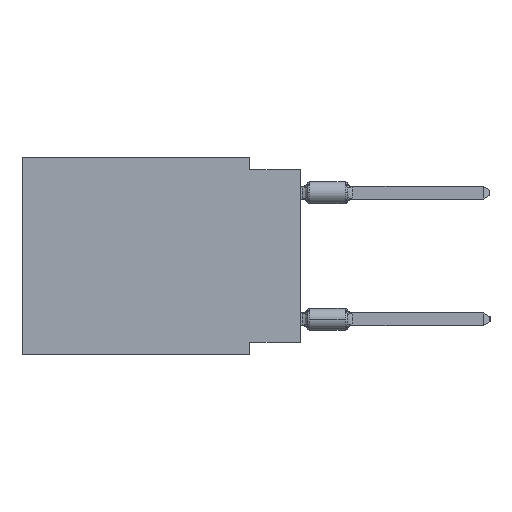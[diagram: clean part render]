
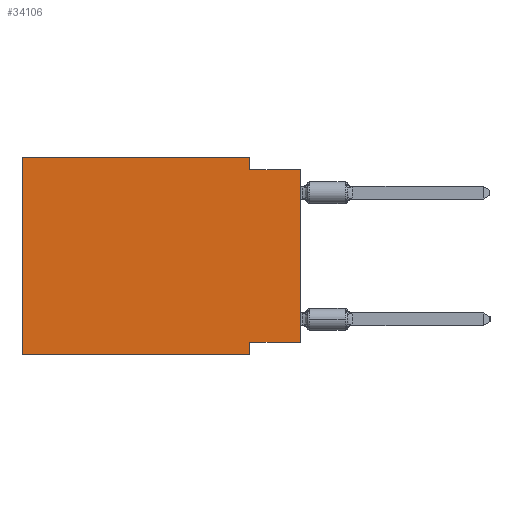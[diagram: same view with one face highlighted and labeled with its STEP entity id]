
A CAD part, left-side view. The second image highlights one B-rep face of the part: STEP entity #34106.
In plain terms, the highlighted planar face has unit normal (-1, 0, 0).
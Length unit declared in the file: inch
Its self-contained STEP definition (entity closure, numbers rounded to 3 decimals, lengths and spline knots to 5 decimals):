
#138 = EDGE_CURVE ( 'NONE', #9546, #27398, #3173, .T. ) ;
#613 = CARTESIAN_POINT ( 'NONE',  ( 0., 0., -0.365 ) ) ;
#2418 = DIRECTION ( 'NONE',  ( 0., 0., -1. ) ) ;
#2647 = EDGE_CURVE ( 'NONE', #13642, #23182, #25078, .T. ) ;
#2882 = CARTESIAN_POINT ( 'NONE',  ( 0., 0.55, 0. ) ) ;
#3173 = LINE ( 'NONE', #27430, #21634 ) ;
#3819 = DIRECTION ( 'NONE',  ( 0., -1., 0. ) ) ;
#4857 = DIRECTION ( 'NONE',  ( 0., -1., 0. ) ) ;
#7049 = LINE ( 'NONE', #25721, #18120 ) ;
#7092 = VECTOR ( 'NONE', #3819, 39.37008 ) ;
#7544 = VERTEX_POINT ( 'NONE', #15903 ) ;
#7547 = CARTESIAN_POINT ( 'NONE',  ( 0., 0.1, -0.39 ) ) ;
#7665 = LINE ( 'NONE', #9941, #9378 ) ;
#8382 = ORIENTED_EDGE ( 'NONE', *, *, #31932, .F. ) ;
#8391 = LINE ( 'NONE', #38871, #14001 ) ;
#8709 = DIRECTION ( 'NONE',  ( 0., -1., 0. ) ) ;
#8732 = ORIENTED_EDGE ( 'NONE', *, *, #20691, .T. ) ;
#9378 = VECTOR ( 'NONE', #4857, 39.37008 ) ;
#9546 = VERTEX_POINT ( 'NONE', #613 ) ;
#9941 = CARTESIAN_POINT ( 'NONE',  ( 0., 0., -0.025 ) ) ;
#10031 = AXIS2_PLACEMENT_3D ( 'NONE', #22576, #34828, #31801 ) ;
#10983 = EDGE_CURVE ( 'NONE', #38676, #13642, #21700, .T. ) ;
#11616 = CARTESIAN_POINT ( 'NONE',  ( 0., 0.1, -0.39 ) ) ;
#12062 = CARTESIAN_POINT ( 'NONE',  ( 0., 0.55, 0. ) ) ;
#12596 = CARTESIAN_POINT ( 'NONE',  ( 0., 0., -0.025 ) ) ;
#12667 = DIRECTION ( 'NONE',  ( 0., 0., 1. ) ) ;
#12937 = ORIENTED_EDGE ( 'NONE', *, *, #2647, .F. ) ;
#13146 = PLANE ( 'NONE',  #10031 ) ;
#13642 = VERTEX_POINT ( 'NONE', #2882 ) ;
#14001 = VECTOR ( 'NONE', #14604, 39.37008 ) ;
#14604 = DIRECTION ( 'NONE',  ( 0., 0., -1. ) ) ;
#15395 = DIRECTION ( 'NONE',  ( 0., 1., 0. ) ) ;
#15903 = CARTESIAN_POINT ( 'NONE',  ( 0., 0.1, -0.025 ) ) ;
#16757 = FACE_OUTER_BOUND ( 'NONE', #26975, .T. ) ;
#17023 = EDGE_CURVE ( 'NONE', #27398, #38483, #38894, .T. ) ;
#18120 = VECTOR ( 'NONE', #25914, 39.37008 ) ;
#19517 = CARTESIAN_POINT ( 'NONE',  ( 0., 0.1, 0. ) ) ;
#20691 = EDGE_CURVE ( 'NONE', #9546, #32707, #7049, .T. ) ;
#20730 = VECTOR ( 'NONE', #8709, 39.37008 ) ;
#21634 = VECTOR ( 'NONE', #15395, 39.37008 ) ;
#21700 = LINE ( 'NONE', #12062, #23670 ) ;
#21729 = EDGE_CURVE ( 'NONE', #38676, #38483, #39206, .T. ) ;
#21929 = ORIENTED_EDGE ( 'NONE', *, *, #25494, .F. ) ;
#22576 = CARTESIAN_POINT ( 'NONE',  ( 0., 0.55, 0. ) ) ;
#23182 = VERTEX_POINT ( 'NONE', #19517 ) ;
#23670 = VECTOR ( 'NONE', #12667, 39.37008 ) ;
#24360 = CARTESIAN_POINT ( 'NONE',  ( 0., 0.55, -0.39 ) ) ;
#24650 = ORIENTED_EDGE ( 'NONE', *, *, #10983, .F. ) ;
#25078 = LINE ( 'NONE', #28303, #7092 ) ;
#25494 = EDGE_CURVE ( 'NONE', #23182, #7544, #8391, .T. ) ;
#25721 = CARTESIAN_POINT ( 'NONE',  ( 0., 0., 0. ) ) ;
#25914 = DIRECTION ( 'NONE',  ( 0., 0., 1. ) ) ;
#26975 = EDGE_LOOP ( 'NONE', ( #8732, #8382, #21929, #12937, #24650, #29698, #34787, #27112 ) ) ;
#27112 = ORIENTED_EDGE ( 'NONE', *, *, #138, .F. ) ;
#27398 = VERTEX_POINT ( 'NONE', #31279 ) ;
#27430 = CARTESIAN_POINT ( 'NONE',  ( 0., 0., -0.365 ) ) ;
#28303 = CARTESIAN_POINT ( 'NONE',  ( 0., 0.55, 0. ) ) ;
#29698 = ORIENTED_EDGE ( 'NONE', *, *, #21729, .T. ) ;
#31279 = CARTESIAN_POINT ( 'NONE',  ( 0., 0.1, -0.365 ) ) ;
#31801 = DIRECTION ( 'NONE',  ( 0., 0., -1. ) ) ;
#31932 = EDGE_CURVE ( 'NONE', #7544, #32707, #7665, .T. ) ;
#32707 = VERTEX_POINT ( 'NONE', #12596 ) ;
#32754 = VECTOR ( 'NONE', #2418, 39.37008 ) ;
#34106 = ADVANCED_FACE ( 'NONE', ( #16757 ), #13146, .F. ) ;
#34787 = ORIENTED_EDGE ( 'NONE', *, *, #17023, .F. ) ;
#34828 = DIRECTION ( 'NONE',  ( 1., 0., 0. ) ) ;
#36215 = CARTESIAN_POINT ( 'NONE',  ( 0., 0.55, -0.39 ) ) ;
#38483 = VERTEX_POINT ( 'NONE', #7547 ) ;
#38676 = VERTEX_POINT ( 'NONE', #36215 ) ;
#38871 = CARTESIAN_POINT ( 'NONE',  ( 0., 0.1, 0. ) ) ;
#38894 = LINE ( 'NONE', #11616, #32754 ) ;
#39206 = LINE ( 'NONE', #24360, #20730 ) ;
